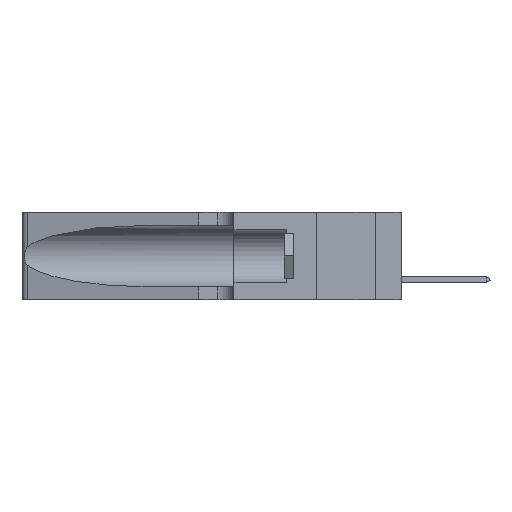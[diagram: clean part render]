
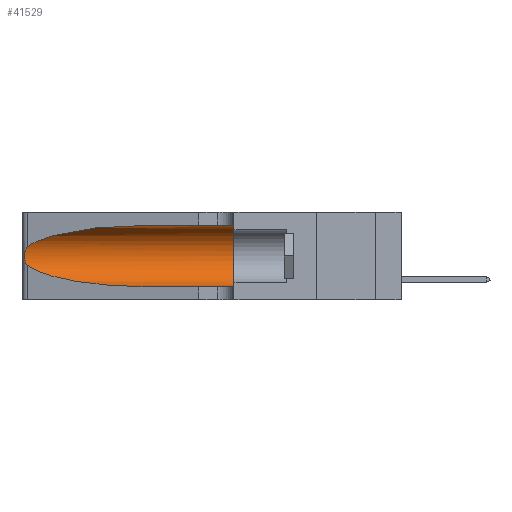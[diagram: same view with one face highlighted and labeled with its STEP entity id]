
A CAD part, left-side view. The second image highlights one B-rep face of the part: STEP entity #41529.
In plain terms, the highlighted cylindrical face has radius 3.308 mm (diameter 6.617 mm), a partial arc.
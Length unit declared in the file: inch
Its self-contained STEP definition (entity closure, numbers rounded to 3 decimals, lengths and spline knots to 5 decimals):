
#1297 = CARTESIAN_POINT ( 'NONE',  ( 0.25487, 1.22718, 0.14631 ) ) ;
#2266 = CARTESIAN_POINT ( 'NONE',  ( 0.26017, 1.23833, 0.17102 ) ) ;
#3501 = CARTESIAN_POINT ( 'NONE',  ( 0.1305, 1.61858, 0.05475 ) ) ;
#3605 = EDGE_CURVE ( 'NONE', #14091, #19248, #8183, .T. ) ;
#3894 = VERTEX_POINT ( 'NONE', #27301 ) ;
#4530 = CARTESIAN_POINT ( 'NONE',  ( 0.25487, 1.22718, 0.22369 ) ) ;
#5224 = VERTEX_POINT ( 'NONE', #41179 ) ;
#5417 = CARTESIAN_POINT ( 'NONE',  ( 0.26018, 1.23835, 0.19895 ) ) ;
#5698 = LINE ( 'NONE', #3501, #15652 ) ;
#6047 = EDGE_CURVE ( 'NONE', #3894, #35226, #42928, .T. ) ;
#6595 = ORIENTED_EDGE ( 'NONE', *, *, #42890, .T. ) ;
#6964 = DIRECTION ( 'NONE',  ( 0., -1., 0. ) ) ;
#7298 = CARTESIAN_POINT ( 'NONE',  ( 0.1305, 1.61858, 0.185 ) ) ;
#7841 = CARTESIAN_POINT ( 'NONE',  ( 0.2373, 1.15595, 0.08982 ) ) ;
#8019 = CARTESIAN_POINT ( 'NONE',  ( 0.1305, 0.72297, 0.05475 ) ) ;
#8183 = LINE ( 'NONE', #12104, #40472 ) ;
#8431 = CARTESIAN_POINT ( 'NONE',  ( 0.1305, 0.72297, 0.05475 ) ) ;
#8496 =( BOUNDED_CURVE ( )  B_SPLINE_CURVE ( 3, ( #14370, #34543, #41280, #10727 ),
 .UNSPECIFIED., .F., .F. ) 
 B_SPLINE_CURVE_WITH_KNOTS ( ( 4, 4 ),
 ( 1.5708, 2.84003 ),
 .UNSPECIFIED. ) 
 CURVE ( )  GEOMETRIC_REPRESENTATION_ITEM ( )  RATIONAL_B_SPLINE_CURVE ( ( 1., 0.87, 0.87, 1. ) ) 
 REPRESENTATION_ITEM ( '' )  );
#10727 = CARTESIAN_POINT ( 'NONE',  ( 0.25487, 1.22718, 0.22369 ) ) ;
#12104 = CARTESIAN_POINT ( 'NONE',  ( 0.1305, 1.61858, 0.31525 ) ) ;
#12303 = CARTESIAN_POINT ( 'NONE',  ( 0.25487, 1.22718, 0.22369 ) ) ;
#12681 = EDGE_CURVE ( 'NONE', #13449, #3894, #29842, .T. ) ;
#13154 = ORIENTED_EDGE ( 'NONE', *, *, #3605, .F. ) ;
#13449 = VERTEX_POINT ( 'NONE', #4530 ) ;
#14091 = VERTEX_POINT ( 'NONE', #19214 ) ;
#14172 = DIRECTION ( 'NONE',  ( 0., 0., -1. ) ) ;
#14370 = CARTESIAN_POINT ( 'NONE',  ( 0.1305, 0.72297, 0.31525 ) ) ;
#14817 = CIRCLE ( 'NONE', #19824, 0.13025 ) ;
#15469 = DIRECTION ( 'NONE',  ( 0., -1., 0. ) ) ;
#15652 = VECTOR ( 'NONE', #6964, 39.37008 ) ;
#15671 = CARTESIAN_POINT ( 'NONE',  ( 0.25487, 1.22718, 0.14631 ) ) ;
#15820 = CARTESIAN_POINT ( 'NONE',  ( 0.25555, 1.22993, 0.14849 ) ) ;
#15958 = CARTESIAN_POINT ( 'NONE',  ( 0.25787, 1.23484, 0.2124 ) ) ;
#17504 = CYLINDRICAL_SURFACE ( 'NONE', #35022, 0.13025 ) ;
#17920 = CARTESIAN_POINT ( 'NONE',  ( 0.1305, 0.35, 0.185 ) ) ;
#18857 = CARTESIAN_POINT ( 'NONE',  ( 0.25854, 1.2359, 0.20912 ) ) ;
#19214 = CARTESIAN_POINT ( 'NONE',  ( 0.1305, 0.72297, 0.31525 ) ) ;
#19248 = VERTEX_POINT ( 'NONE', #25605 ) ;
#19824 = AXIS2_PLACEMENT_3D ( 'NONE', #17920, #41380, #21418 ) ;
#20723 = DIRECTION ( 'NONE',  ( 0., -1., 0. ) ) ;
#21386 = FACE_OUTER_BOUND ( 'NONE', #26415, .T. ) ;
#21418 = DIRECTION ( 'NONE',  ( 0., 0., 1. ) ) ;
#22252 = ORIENTED_EDGE ( 'NONE', *, *, #35138, .F. ) ;
#22605 = CARTESIAN_POINT ( 'NONE',  ( 0.26075, 1.23896, 0.19203 ) ) ;
#25605 = CARTESIAN_POINT ( 'NONE',  ( 0.1305, 0.35, 0.31525 ) ) ;
#25857 = CARTESIAN_POINT ( 'NONE',  ( 0.26075, 1.23896, 0.178 ) ) ;
#26415 = EDGE_LOOP ( 'NONE', ( #6595, #36611, #41702, #30702, #22252, #13154 ) ) ;
#27301 = CARTESIAN_POINT ( 'NONE',  ( 0.25487, 1.22718, 0.14631 ) ) ;
#28815 = CARTESIAN_POINT ( 'NONE',  ( 0.18966, 0.96281, 0.05475 ) ) ;
#29036 = CARTESIAN_POINT ( 'NONE',  ( 0.25639, 1.23184, 0.21858 ) ) ;
#29842 = B_SPLINE_CURVE_WITH_KNOTS ( 'NONE', 3,
 ( #12303, #35257, #29036, #15958, #18857, #5417, #22605, #25857, #2266, #35533, #35818, #39207, #15820, #15671 ),
 .UNSPECIFIED., .F., .F.,
 ( 4, 2, 2, 2, 2, 2, 4 ),
 ( 0., 0.00027, 0.00053, 0.00107, 0.0016, 0.00187, 0.00214 ),
 .UNSPECIFIED. ) ;
#30702 = ORIENTED_EDGE ( 'NONE', *, *, #37136, .T. ) ;
#34543 = CARTESIAN_POINT ( 'NONE',  ( 0.18966, 0.96281, 0.31525 ) ) ;
#35022 = AXIS2_PLACEMENT_3D ( 'NONE', #7298, #20723, #14172 ) ;
#35138 = EDGE_CURVE ( 'NONE', #19248, #5224, #14817, .T. ) ;
#35226 = VERTEX_POINT ( 'NONE', #8019 ) ;
#35257 = CARTESIAN_POINT ( 'NONE',  ( 0.25555, 1.22994, 0.2215 ) ) ;
#35533 = CARTESIAN_POINT ( 'NONE',  ( 0.25856, 1.23593, 0.16098 ) ) ;
#35818 = CARTESIAN_POINT ( 'NONE',  ( 0.25789, 1.23486, 0.15765 ) ) ;
#36611 = ORIENTED_EDGE ( 'NONE', *, *, #12681, .T. ) ;
#37136 = EDGE_CURVE ( 'NONE', #35226, #5224, #5698, .T. ) ;
#39207 = CARTESIAN_POINT ( 'NONE',  ( 0.25639, 1.23186, 0.15144 ) ) ;
#40472 = VECTOR ( 'NONE', #15469, 39.37008 ) ;
#41179 = CARTESIAN_POINT ( 'NONE',  ( 0.1305, 0.35, 0.05475 ) ) ;
#41280 = CARTESIAN_POINT ( 'NONE',  ( 0.2373, 1.15595, 0.28018 ) ) ;
#41380 = DIRECTION ( 'NONE',  ( 0., 1., 0. ) ) ;
#41529 = ADVANCED_FACE ( 'NONE', ( #21386 ), #17504, .F. ) ;
#41702 = ORIENTED_EDGE ( 'NONE', *, *, #6047, .T. ) ;
#42890 = EDGE_CURVE ( 'NONE', #14091, #13449, #8496, .T. ) ;
#42928 =( BOUNDED_CURVE ( )  B_SPLINE_CURVE ( 3, ( #1297, #7841, #28815, #8431 ),
 .UNSPECIFIED., .F., .T. ) 
 B_SPLINE_CURVE_WITH_KNOTS ( ( 4, 4 ),
 ( 3.44316, 4.71239 ),
 .UNSPECIFIED. ) 
 CURVE ( )  GEOMETRIC_REPRESENTATION_ITEM ( )  RATIONAL_B_SPLINE_CURVE ( ( 1., 0.87, 0.87, 1. ) ) 
 REPRESENTATION_ITEM ( '' )  );
